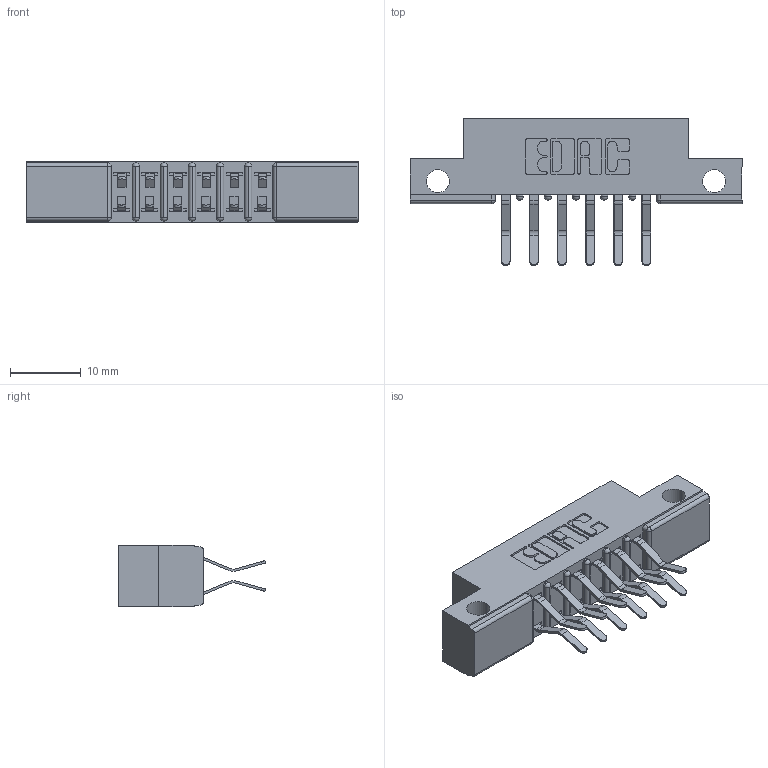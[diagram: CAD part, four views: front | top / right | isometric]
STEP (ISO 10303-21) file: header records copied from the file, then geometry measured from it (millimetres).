
FILE_DESCRIPTION (( 'STEP AP203' ), '1' );
FILE_NAME ('307-012-460-212.STEP', '2020-09-28T15:18:05', ( '' ), ( '' ), 'SwSTEP 2.0', 'SolidWorks 2020', '' );
FILE_SCHEMA (( 'CONFIG_CONTROL_DESIGN' ));
Length unit declared in the file: inch
Products named in the file (3): 307-290-001_560; 307 Part_.128 Dia Side Mounting Holes; 307-012-460-212
Assembly tree (13 placements, depth 2):
  307-012-460-212
    307 Part_.128 Dia Side Mounting Holes
    307-290-001_560  x12
Bounding box: 46.79 x 20.73 x 8.71 mm (x, y, z)
Volume: 3001.2 mm3; surface area: 4419 mm2
Topology: 13 solids, 13 shells, 725 faces, 2027 edges, 1314 vertices
Faces by surface type: plane 466, cylinder 245, sphere 14
Entity records: 9880 total; most frequent: CARTESIAN_POINT 1626, DIRECTION 1609, ORIENTED_EDGE 1606, EDGE_CURVE 803, LINE 599, VECTOR 599, VERTEX_POINT 522, AXIS2_PLACEMENT_3D 505
